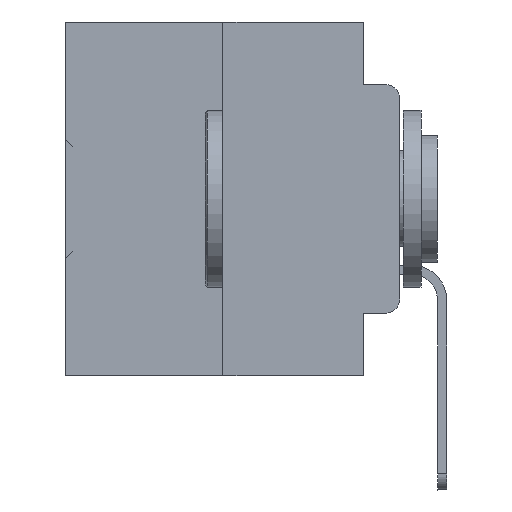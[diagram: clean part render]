
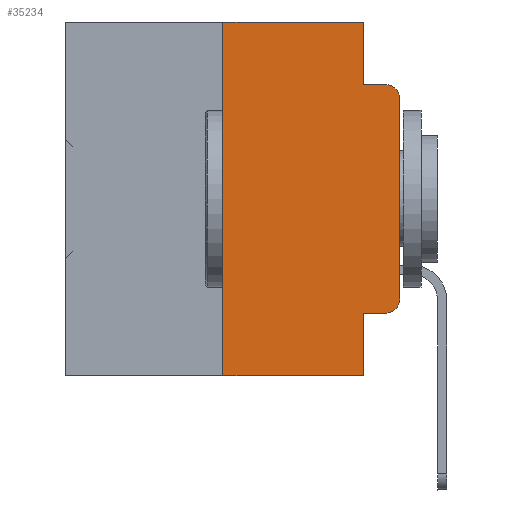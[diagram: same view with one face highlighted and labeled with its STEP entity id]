
A CAD part, left-side view. The second image highlights one B-rep face of the part: STEP entity #35234.
In plain terms, the highlighted planar face has unit normal (-1, 0, 0).
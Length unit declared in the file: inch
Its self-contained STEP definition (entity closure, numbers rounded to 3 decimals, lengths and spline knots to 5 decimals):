
#469 = DIRECTION ( 'NONE',  ( 1., 0., 0. ) ) ;
#1300 = EDGE_CURVE ( 'NONE', #34959, #18017, #11937, .T. ) ;
#2103 = VECTOR ( 'NONE', #11826, 39.37008 ) ;
#2466 = EDGE_CURVE ( 'NONE', #12560, #25678, #21798, .T. ) ;
#2838 = CARTESIAN_POINT ( 'NONE',  ( 0., 0., -0.1085 ) ) ;
#3640 = CARTESIAN_POINT ( 'NONE',  ( 0., 0.051, 0. ) ) ;
#3922 = ORIENTED_EDGE ( 'NONE', *, *, #21996, .T. ) ;
#4270 = CARTESIAN_POINT ( 'NONE',  ( 0., 0.25, -0.5 ) ) ;
#4363 = LINE ( 'NONE', #16278, #35573 ) ;
#4395 = DIRECTION ( 'NONE',  ( 0., 0., -1. ) ) ;
#4661 = DIRECTION ( 'NONE',  ( 0., -1., 0. ) ) ;
#5180 = CARTESIAN_POINT ( 'NONE',  ( 0., 0.02, -0.3915 ) ) ;
#5432 = LINE ( 'NONE', #38078, #17612 ) ;
#5675 = ORIENTED_EDGE ( 'NONE', *, *, #18461, .F. ) ;
#5884 = AXIS2_PLACEMENT_3D ( 'NONE', #31732, #28801, #22557 ) ;
#6188 = EDGE_CURVE ( 'NONE', #28056, #15090, #30061, .T. ) ;
#6199 = ORIENTED_EDGE ( 'NONE', *, *, #12237, .F. ) ;
#6716 = DIRECTION ( 'NONE',  ( 0., 0., -1. ) ) ;
#7245 = LINE ( 'NONE', #19150, #24826 ) ;
#7481 = DIRECTION ( 'NONE',  ( 0., -1., 0. ) ) ;
#7588 = AXIS2_PLACEMENT_3D ( 'NONE', #5180, #29000, #4395 ) ;
#7699 = EDGE_CURVE ( 'NONE', #25678, #28056, #5432, .T. ) ;
#7846 = CARTESIAN_POINT ( 'NONE',  ( 0., 0.051, -0.5 ) ) ;
#9260 = PLANE ( 'NONE',  #22765 ) ;
#9823 = CARTESIAN_POINT ( 'NONE',  ( 0., 0.25, 0. ) ) ;
#10062 = CARTESIAN_POINT ( 'NONE',  ( 0., 0.25, 0. ) ) ;
#10882 = EDGE_CURVE ( 'NONE', #20048, #34959, #7245, .T. ) ;
#11549 = ORIENTED_EDGE ( 'NONE', *, *, #24670, .T. ) ;
#11805 = FACE_OUTER_BOUND ( 'NONE', #29461, .T. ) ;
#11826 = DIRECTION ( 'NONE',  ( 0., 0., 1. ) ) ;
#11937 = CIRCLE ( 'NONE', #7588, 0.02 ) ;
#12237 = EDGE_CURVE ( 'NONE', #15090, #28558, #4363, .T. ) ;
#12536 = ORIENTED_EDGE ( 'NONE', *, *, #32751, .T. ) ;
#12560 = VERTEX_POINT ( 'NONE', #4270 ) ;
#13373 = VERTEX_POINT ( 'NONE', #2838 ) ;
#14030 = LINE ( 'NONE', #38070, #14053 ) ;
#14053 = VECTOR ( 'NONE', #31787, 39.37008 ) ;
#14717 = ORIENTED_EDGE ( 'NONE', *, *, #1300, .T. ) ;
#15090 = VERTEX_POINT ( 'NONE', #21298 ) ;
#15547 = CARTESIAN_POINT ( 'NONE',  ( 0., 0.051, 0. ) ) ;
#16278 = CARTESIAN_POINT ( 'NONE',  ( 0., 0.051, -0.0885 ) ) ;
#17483 = LINE ( 'NONE', #38626, #2103 ) ;
#17612 = VECTOR ( 'NONE', #4661, 39.37008 ) ;
#18017 = VERTEX_POINT ( 'NONE', #28092 ) ;
#18461 = EDGE_CURVE ( 'NONE', #20048, #38439, #30407, .T. ) ;
#19150 = CARTESIAN_POINT ( 'NONE',  ( 0., 0.051, -0.4115 ) ) ;
#19937 = ORIENTED_EDGE ( 'NONE', *, *, #10882, .T. ) ;
#20048 = VERTEX_POINT ( 'NONE', #33517 ) ;
#20887 = DIRECTION ( 'NONE',  ( 0., 0., -1. ) ) ;
#21298 = CARTESIAN_POINT ( 'NONE',  ( 0., 0.051, -0.0885 ) ) ;
#21798 = LINE ( 'NONE', #10062, #22609 ) ;
#21996 = EDGE_CURVE ( 'NONE', #13373, #28558, #30826, .T. ) ;
#22519 = VECTOR ( 'NONE', #27464, 39.37008 ) ;
#22557 = DIRECTION ( 'NONE',  ( 0., 0., -1. ) ) ;
#22609 = VECTOR ( 'NONE', #33727, 39.37008 ) ;
#22765 = AXIS2_PLACEMENT_3D ( 'NONE', #27420, #469, #6716 ) ;
#23501 = VECTOR ( 'NONE', #20887, 39.37008 ) ;
#24194 = CARTESIAN_POINT ( 'NONE',  ( 0., 0.051, 0. ) ) ;
#24670 = EDGE_CURVE ( 'NONE', #12560, #38439, #14030, .T. ) ;
#24826 = VECTOR ( 'NONE', #25586, 39.37008 ) ;
#25586 = DIRECTION ( 'NONE',  ( 0., -1., 0. ) ) ;
#25678 = VERTEX_POINT ( 'NONE', #9823 ) ;
#27166 = ORIENTED_EDGE ( 'NONE', *, *, #6188, .F. ) ;
#27420 = CARTESIAN_POINT ( 'NONE',  ( 0., 0.473, 0. ) ) ;
#27464 = DIRECTION ( 'NONE',  ( 0., 0., -1. ) ) ;
#28056 = VERTEX_POINT ( 'NONE', #15547 ) ;
#28092 = CARTESIAN_POINT ( 'NONE',  ( 0., 0., -0.3915 ) ) ;
#28558 = VERTEX_POINT ( 'NONE', #33685 ) ;
#28801 = DIRECTION ( 'NONE',  ( -1., 0., 0. ) ) ;
#29000 = DIRECTION ( 'NONE',  ( -1., 0., 0. ) ) ;
#29461 = EDGE_LOOP ( 'NONE', ( #12536, #3922, #6199, #27166, #29664, #35554, #11549, #5675, #19937, #14717 ) ) ;
#29664 = ORIENTED_EDGE ( 'NONE', *, *, #7699, .F. ) ;
#30061 = LINE ( 'NONE', #24194, #23501 ) ;
#30407 = LINE ( 'NONE', #3640, #22519 ) ;
#30449 = CARTESIAN_POINT ( 'NONE',  ( 0., 0.02, -0.4115 ) ) ;
#30826 = CIRCLE ( 'NONE', #5884, 0.02 ) ;
#31732 = CARTESIAN_POINT ( 'NONE',  ( 0., 0.02, -0.1085 ) ) ;
#31787 = DIRECTION ( 'NONE',  ( 0., -1., 0. ) ) ;
#32751 = EDGE_CURVE ( 'NONE', #18017, #13373, #17483, .T. ) ;
#33517 = CARTESIAN_POINT ( 'NONE',  ( 0., 0.051, -0.4115 ) ) ;
#33685 = CARTESIAN_POINT ( 'NONE',  ( 0., 0.02, -0.0885 ) ) ;
#33727 = DIRECTION ( 'NONE',  ( 0., 0., 1. ) ) ;
#34959 = VERTEX_POINT ( 'NONE', #30449 ) ;
#35234 = ADVANCED_FACE ( 'NONE', ( #11805 ), #9260, .F. ) ;
#35554 = ORIENTED_EDGE ( 'NONE', *, *, #2466, .F. ) ;
#35573 = VECTOR ( 'NONE', #7481, 39.37008 ) ;
#38070 = CARTESIAN_POINT ( 'NONE',  ( 0., 0.473, -0.5 ) ) ;
#38078 = CARTESIAN_POINT ( 'NONE',  ( 0., 0.473, 0. ) ) ;
#38439 = VERTEX_POINT ( 'NONE', #7846 ) ;
#38626 = CARTESIAN_POINT ( 'NONE',  ( 0., 0., 0. ) ) ;
